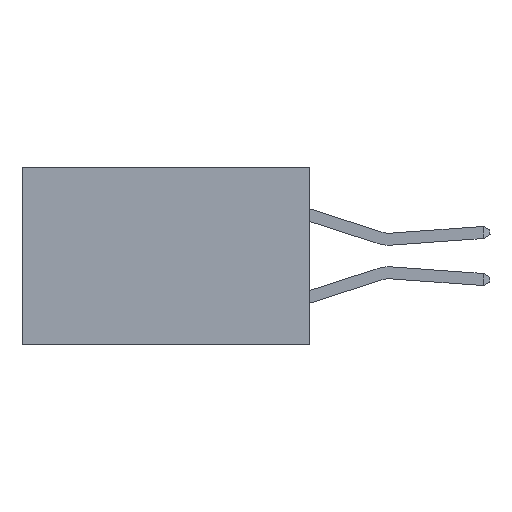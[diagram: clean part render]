
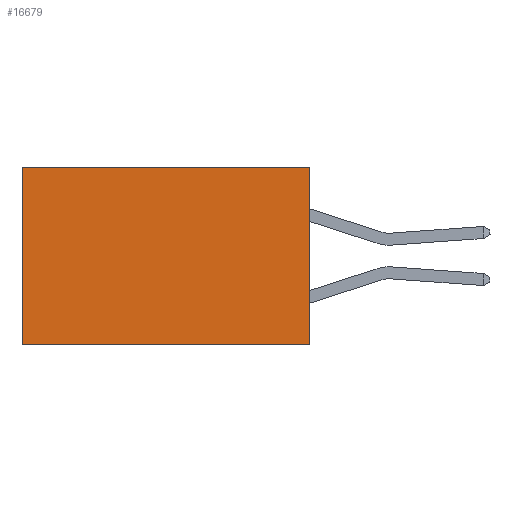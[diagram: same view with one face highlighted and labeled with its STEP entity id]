
A CAD part, left-side view. The second image highlights one B-rep face of the part: STEP entity #16679.
In plain terms, the highlighted planar face has unit normal (-1, 0, 0).
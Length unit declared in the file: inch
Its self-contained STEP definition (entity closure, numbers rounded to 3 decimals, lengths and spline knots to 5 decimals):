
#1710 = LINE ( 'NONE', #18312, #6673 ) ;
#2049 = DIRECTION ( 'NONE',  ( 1., 0., 0. ) ) ;
#2994 = DIRECTION ( 'NONE',  ( 0., 1., 0. ) ) ;
#5340 = EDGE_CURVE ( 'NONE', #6578, #17490, #19755, .T. ) ;
#6376 = ORIENTED_EDGE ( 'NONE', *, *, #12815, .F. ) ;
#6578 = VERTEX_POINT ( 'NONE', #25369 ) ;
#6673 = VECTOR ( 'NONE', #26260, 39.37008 ) ;
#7423 = FACE_OUTER_BOUND ( 'NONE', #9794, .T. ) ;
#8186 = EDGE_CURVE ( 'NONE', #20275, #17490, #1710, .T. ) ;
#8213 = AXIS2_PLACEMENT_3D ( 'NONE', #12319, #2049, #16403 ) ;
#9024 = VECTOR ( 'NONE', #14743, 39.37008 ) ;
#9794 = EDGE_LOOP ( 'NONE', ( #25290, #24552, #6376, #17605 ) ) ;
#11277 = LINE ( 'NONE', #25982, #17261 ) ;
#11926 = CARTESIAN_POINT ( 'NONE',  ( 0.2615, 0.6, 0. ) ) ;
#12121 = CARTESIAN_POINT ( 'NONE',  ( 0.2615, 0., 0. ) ) ;
#12319 = CARTESIAN_POINT ( 'NONE',  ( 0.2615, 0., -0.37 ) ) ;
#12815 = EDGE_CURVE ( 'NONE', #17326, #6578, #11277, .T. ) ;
#14618 = CARTESIAN_POINT ( 'NONE',  ( 0.2615, 0., -0.37 ) ) ;
#14743 = DIRECTION ( 'NONE',  ( 0., 1., 0. ) ) ;
#15295 = CARTESIAN_POINT ( 'NONE',  ( 0.2615, 0., 0. ) ) ;
#15945 = DIRECTION ( 'NONE',  ( 0., 0., -1. ) ) ;
#16403 = DIRECTION ( 'NONE',  ( 0., 0., -1. ) ) ;
#16679 = ADVANCED_FACE ( 'NONE', ( #7423 ), #18324, .F. ) ;
#17261 = VECTOR ( 'NONE', #15945, 39.37008 ) ;
#17326 = VERTEX_POINT ( 'NONE', #12121 ) ;
#17490 = VERTEX_POINT ( 'NONE', #18651 ) ;
#17605 = ORIENTED_EDGE ( 'NONE', *, *, #18638, .T. ) ;
#18312 = CARTESIAN_POINT ( 'NONE',  ( 0.2615, 0.6, -0.37 ) ) ;
#18324 = PLANE ( 'NONE',  #8213 ) ;
#18638 = EDGE_CURVE ( 'NONE', #17326, #20275, #24062, .T. ) ;
#18651 = CARTESIAN_POINT ( 'NONE',  ( 0.2615, 0.6, -0.37 ) ) ;
#19755 = LINE ( 'NONE', #14618, #9024 ) ;
#20275 = VERTEX_POINT ( 'NONE', #11926 ) ;
#24062 = LINE ( 'NONE', #15295, #24679 ) ;
#24552 = ORIENTED_EDGE ( 'NONE', *, *, #5340, .F. ) ;
#24679 = VECTOR ( 'NONE', #2994, 39.37008 ) ;
#25290 = ORIENTED_EDGE ( 'NONE', *, *, #8186, .T. ) ;
#25369 = CARTESIAN_POINT ( 'NONE',  ( 0.2615, 0., -0.37 ) ) ;
#25982 = CARTESIAN_POINT ( 'NONE',  ( 0.2615, 0., -0.37 ) ) ;
#26260 = DIRECTION ( 'NONE',  ( 0., 0., -1. ) ) ;
